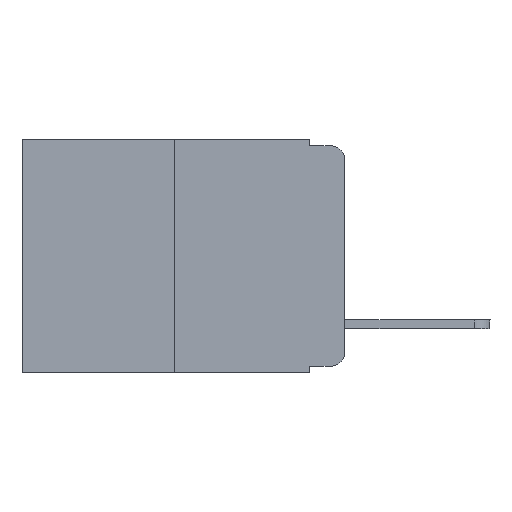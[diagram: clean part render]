
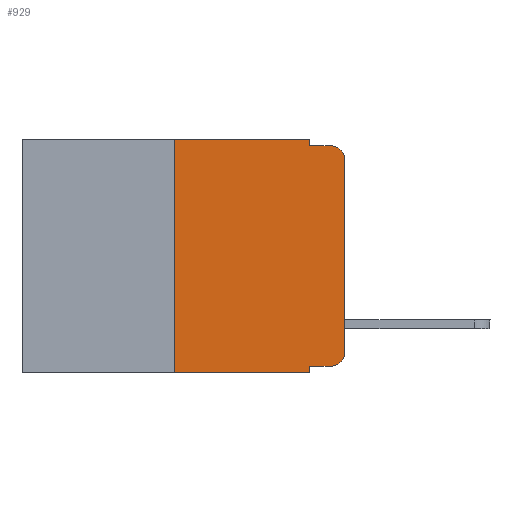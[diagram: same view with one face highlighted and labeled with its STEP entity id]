
A CAD part, left-side view. The second image highlights one B-rep face of the part: STEP entity #929.
In plain terms, the highlighted planar face has unit normal (-1, 0, 0).
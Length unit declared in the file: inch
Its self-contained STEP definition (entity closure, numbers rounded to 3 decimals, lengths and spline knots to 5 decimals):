
#25 = EDGE_CURVE ( 'NONE', #5844, #13552, #2592, .T. ) ;
#37 = ORIENTED_EDGE ( 'NONE', *, *, #5594, .F. ) ;
#630 = CIRCLE ( 'NONE', #3592, 0.02 ) ;
#929 = ADVANCED_FACE ( 'NONE', ( #12855 ), #4530, .F. ) ;
#1118 = VECTOR ( 'NONE', #2110, 39.37008 ) ;
#1224 = LINE ( 'NONE', #14448, #1602 ) ;
#1470 = ORIENTED_EDGE ( 'NONE', *, *, #9545, .T. ) ;
#1588 = CARTESIAN_POINT ( 'NONE',  ( 0., 0.051, -0.01 ) ) ;
#1602 = VECTOR ( 'NONE', #7310, 39.37008 ) ;
#1699 = EDGE_CURVE ( 'NONE', #7173, #13552, #3883, .T. ) ;
#1905 = ORIENTED_EDGE ( 'NONE', *, *, #14758, .F. ) ;
#1914 = LINE ( 'NONE', #6970, #7466 ) ;
#1959 = DIRECTION ( 'NONE',  ( 0., 0., -1. ) ) ;
#2091 = VECTOR ( 'NONE', #11984, 39.37008 ) ;
#2110 = DIRECTION ( 'NONE',  ( 0., 0., -1. ) ) ;
#2215 = EDGE_CURVE ( 'NONE', #9677, #13267, #6084, .T. ) ;
#2241 = DIRECTION ( 'NONE',  ( 0., -1., 0. ) ) ;
#2442 = LINE ( 'NONE', #10909, #2091 ) ;
#2592 = LINE ( 'NONE', #15383, #6693 ) ;
#2684 = ORIENTED_EDGE ( 'NONE', *, *, #6432, .T. ) ;
#2968 = ORIENTED_EDGE ( 'NONE', *, *, #2215, .T. ) ;
#3232 = LINE ( 'NONE', #14496, #13668 ) ;
#3342 = ORIENTED_EDGE ( 'NONE', *, *, #14526, .F. ) ;
#3434 = DIRECTION ( 'NONE',  ( 1., 0., 0. ) ) ;
#3474 = DIRECTION ( 'NONE',  ( 0., -1., 0. ) ) ;
#3533 = ORIENTED_EDGE ( 'NONE', *, *, #25, .T. ) ;
#3592 = AXIS2_PLACEMENT_3D ( 'NONE', #5902, #10741, #3634 ) ;
#3634 = DIRECTION ( 'NONE',  ( 0., 0., -1. ) ) ;
#3883 = LINE ( 'NONE', #9261, #1118 ) ;
#4470 = CARTESIAN_POINT ( 'NONE',  ( 0., 0.051, -0.01 ) ) ;
#4530 = PLANE ( 'NONE',  #12299 ) ;
#4790 = VERTEX_POINT ( 'NONE', #5241 ) ;
#5214 = CARTESIAN_POINT ( 'NONE',  ( 0., 0., -0.313 ) ) ;
#5241 = CARTESIAN_POINT ( 'NONE',  ( 0., 0.25, 0. ) ) ;
#5282 = VERTEX_POINT ( 'NONE', #8188 ) ;
#5594 = EDGE_CURVE ( 'NONE', #5282, #6331, #13289, .T. ) ;
#5844 = VERTEX_POINT ( 'NONE', #11853 ) ;
#5902 = CARTESIAN_POINT ( 'NONE',  ( 0., 0.02, -0.03 ) ) ;
#6032 = ORIENTED_EDGE ( 'NONE', *, *, #13521, .F. ) ;
#6042 = EDGE_CURVE ( 'NONE', #15133, #11295, #630, .T. ) ;
#6084 = CIRCLE ( 'NONE', #11826, 0.02 ) ;
#6331 = VERTEX_POINT ( 'NONE', #4470 ) ;
#6432 = EDGE_CURVE ( 'NONE', #7173, #9677, #1914, .T. ) ;
#6693 = VECTOR ( 'NONE', #3474, 39.37008 ) ;
#6970 = CARTESIAN_POINT ( 'NONE',  ( 0., 0.051, -0.333 ) ) ;
#7173 = VERTEX_POINT ( 'NONE', #11717 ) ;
#7226 = DIRECTION ( 'NONE',  ( 0., 0., -1. ) ) ;
#7310 = DIRECTION ( 'NONE',  ( 0., 0., 1. ) ) ;
#7466 = VECTOR ( 'NONE', #2241, 39.37008 ) ;
#7670 = CARTESIAN_POINT ( 'NONE',  ( 0., 0.02, -0.333 ) ) ;
#7688 = VECTOR ( 'NONE', #8588, 39.37008 ) ;
#8152 = CARTESIAN_POINT ( 'NONE',  ( 0., 0.473, 0. ) ) ;
#8188 = CARTESIAN_POINT ( 'NONE',  ( 0., 0.051, 0. ) ) ;
#8214 = EDGE_LOOP ( 'NONE', ( #1470, #13733, #1905, #37, #3342, #6032, #3533, #9961, #2684, #2968 ) ) ;
#8588 = DIRECTION ( 'NONE',  ( 0., 0., -1. ) ) ;
#9261 = CARTESIAN_POINT ( 'NONE',  ( 0., 0.051, 0. ) ) ;
#9485 = CARTESIAN_POINT ( 'NONE',  ( 0., 0., -0.03 ) ) ;
#9516 = CARTESIAN_POINT ( 'NONE',  ( 0., 0.02, -0.01 ) ) ;
#9545 = EDGE_CURVE ( 'NONE', #13267, #15133, #1224, .T. ) ;
#9677 = VERTEX_POINT ( 'NONE', #7670 ) ;
#9961 = ORIENTED_EDGE ( 'NONE', *, *, #1699, .F. ) ;
#10741 = DIRECTION ( 'NONE',  ( -1., 0., 0. ) ) ;
#10909 = CARTESIAN_POINT ( 'NONE',  ( 0., 0.473, 0. ) ) ;
#11295 = VERTEX_POINT ( 'NONE', #9516 ) ;
#11342 = DIRECTION ( 'NONE',  ( -1., 0., 0. ) ) ;
#11658 = CARTESIAN_POINT ( 'NONE',  ( 0., 0.051, 0. ) ) ;
#11717 = CARTESIAN_POINT ( 'NONE',  ( 0., 0.051, -0.333 ) ) ;
#11826 = AXIS2_PLACEMENT_3D ( 'NONE', #14997, #11342, #1959 ) ;
#11853 = CARTESIAN_POINT ( 'NONE',  ( 0., 0.25, -0.343 ) ) ;
#11984 = DIRECTION ( 'NONE',  ( 0., -1., 0. ) ) ;
#12299 = AXIS2_PLACEMENT_3D ( 'NONE', #8152, #3434, #7226 ) ;
#12696 = VECTOR ( 'NONE', #14985, 39.37008 ) ;
#12855 = FACE_OUTER_BOUND ( 'NONE', #8214, .T. ) ;
#13267 = VERTEX_POINT ( 'NONE', #5214 ) ;
#13289 = LINE ( 'NONE', #11658, #7688 ) ;
#13521 = EDGE_CURVE ( 'NONE', #5844, #4790, #3232, .T. ) ;
#13552 = VERTEX_POINT ( 'NONE', #14544 ) ;
#13616 = LINE ( 'NONE', #1588, #12696 ) ;
#13668 = VECTOR ( 'NONE', #14597, 39.37008 ) ;
#13733 = ORIENTED_EDGE ( 'NONE', *, *, #6042, .T. ) ;
#14448 = CARTESIAN_POINT ( 'NONE',  ( 0., 0., 0. ) ) ;
#14496 = CARTESIAN_POINT ( 'NONE',  ( 0., 0.25, 0. ) ) ;
#14526 = EDGE_CURVE ( 'NONE', #4790, #5282, #2442, .T. ) ;
#14544 = CARTESIAN_POINT ( 'NONE',  ( 0., 0.051, -0.343 ) ) ;
#14597 = DIRECTION ( 'NONE',  ( 0., 0., 1. ) ) ;
#14758 = EDGE_CURVE ( 'NONE', #6331, #11295, #13616, .T. ) ;
#14985 = DIRECTION ( 'NONE',  ( 0., -1., 0. ) ) ;
#14997 = CARTESIAN_POINT ( 'NONE',  ( 0., 0.02, -0.313 ) ) ;
#15133 = VERTEX_POINT ( 'NONE', #9485 ) ;
#15383 = CARTESIAN_POINT ( 'NONE',  ( 0., 0.473, -0.343 ) ) ;
